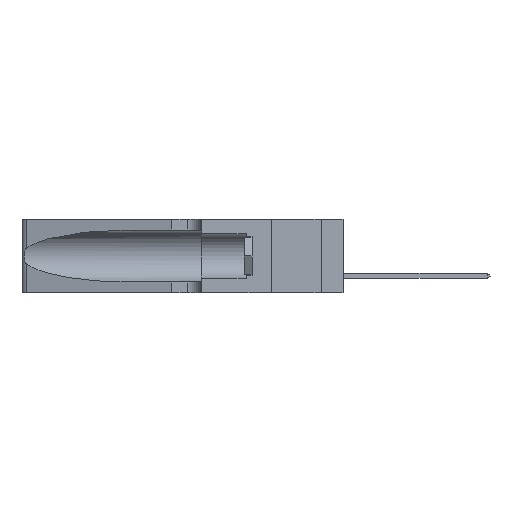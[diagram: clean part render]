
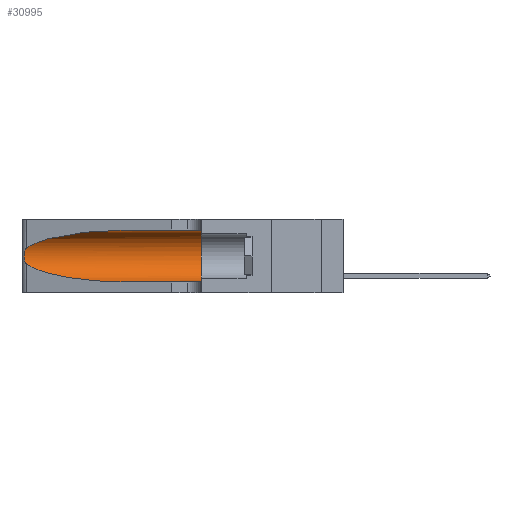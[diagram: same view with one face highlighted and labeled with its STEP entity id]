
A CAD part, left-side view. The second image highlights one B-rep face of the part: STEP entity #30995.
In plain terms, the highlighted cylindrical face has radius 3.308 mm (diameter 6.617 mm), a partial arc.
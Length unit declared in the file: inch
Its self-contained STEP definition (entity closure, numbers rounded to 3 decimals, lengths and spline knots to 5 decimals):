
#220 = CARTESIAN_POINT ( 'NONE',  ( 0.25487, 1.22718, 0.22369 ) ) ;
#691 = CARTESIAN_POINT ( 'NONE',  ( 0.1305, 0.35, 0.185 ) ) ;
#821 = CARTESIAN_POINT ( 'NONE',  ( 0.25789, 1.23486, 0.15765 ) ) ;
#1298 = CARTESIAN_POINT ( 'NONE',  ( 0.25487, 1.22718, 0.14631 ) ) ;
#1674 = CARTESIAN_POINT ( 'NONE',  ( 0.1305, 0.35, 0.05475 ) ) ;
#2868 = CIRCLE ( 'NONE', #6145, 0.13025 ) ;
#4660 = CARTESIAN_POINT ( 'NONE',  ( 0.25787, 1.23484, 0.2124 ) ) ;
#4814 = CARTESIAN_POINT ( 'NONE',  ( 0.26075, 1.23896, 0.178 ) ) ;
#5688 = VECTOR ( 'NONE', #42577, 39.37008 ) ;
#5845 = EDGE_CURVE ( 'NONE', #40393, #30720, #21798, .T. ) ;
#6107 = CARTESIAN_POINT ( 'NONE',  ( 0.1305, 0.72297, 0.05475 ) ) ;
#6145 = AXIS2_PLACEMENT_3D ( 'NONE', #691, #7439, #26365 ) ;
#6199 = CARTESIAN_POINT ( 'NONE',  ( 0.1305, 1.61858, 0.05475 ) ) ;
#6645 = EDGE_CURVE ( 'NONE', #20027, #35176, #32042, .T. ) ;
#7439 = DIRECTION ( 'NONE',  ( 0., 1., 0. ) ) ;
#8121 = DIRECTION ( 'NONE',  ( 0., 0., -1. ) ) ;
#8337 = ORIENTED_EDGE ( 'NONE', *, *, #5845, .T. ) ;
#8373 = CARTESIAN_POINT ( 'NONE',  ( 0.25639, 1.23184, 0.21858 ) ) ;
#9470 = EDGE_CURVE ( 'NONE', #30720, #21175, #28301, .T. ) ;
#10138 = CARTESIAN_POINT ( 'NONE',  ( 0.25487, 1.22718, 0.14631 ) ) ;
#10263 = EDGE_CURVE ( 'NONE', #20027, #40393, #16214, .T. ) ;
#10413 = EDGE_CURVE ( 'NONE', #35176, #31136, #2868, .T. ) ;
#11972 = DIRECTION ( 'NONE',  ( 0., -1., 0. ) ) ;
#12222 = CARTESIAN_POINT ( 'NONE',  ( 0.26075, 1.23896, 0.19203 ) ) ;
#12375 = CARTESIAN_POINT ( 'NONE',  ( 0.26018, 1.23835, 0.19895 ) ) ;
#13506 = EDGE_LOOP ( 'NONE', ( #20761, #8337, #34533, #29191, #28066, #44213 ) ) ;
#16214 =( BOUNDED_CURVE ( )  B_SPLINE_CURVE ( 3, ( #42742, #20967, #28691, #17423 ),
 .UNSPECIFIED., .F., .F. ) 
 B_SPLINE_CURVE_WITH_KNOTS ( ( 4, 4 ),
 ( 1.5708, 2.84003 ),
 .UNSPECIFIED. ) 
 CURVE ( )  GEOMETRIC_REPRESENTATION_ITEM ( )  RATIONAL_B_SPLINE_CURVE ( ( 1., 0.87, 0.87, 1. ) ) 
 REPRESENTATION_ITEM ( '' )  );
#17225 = CARTESIAN_POINT ( 'NONE',  ( 0.1305, 0.35, 0.31525 ) ) ;
#17423 = CARTESIAN_POINT ( 'NONE',  ( 0.25487, 1.22718, 0.22369 ) ) ;
#17577 = CARTESIAN_POINT ( 'NONE',  ( 0.1305, 0.72297, 0.31525 ) ) ;
#20027 = VERTEX_POINT ( 'NONE', #17577 ) ;
#20554 = CARTESIAN_POINT ( 'NONE',  ( 0.2373, 1.15595, 0.08982 ) ) ;
#20761 = ORIENTED_EDGE ( 'NONE', *, *, #10263, .T. ) ;
#20967 = CARTESIAN_POINT ( 'NONE',  ( 0.18966, 0.96281, 0.31525 ) ) ;
#21175 = VERTEX_POINT ( 'NONE', #41529 ) ;
#21798 = B_SPLINE_CURVE_WITH_KNOTS ( 'NONE', 3,
 ( #23424, #34202, #8373, #4660, #45061, #12375, #12222, #4814, #38177, #26821, #821, #37521, #41678, #1298 ),
 .UNSPECIFIED., .F., .F.,
 ( 4, 2, 2, 2, 2, 2, 4 ),
 ( 0., 0.00027, 0.00053, 0.00107, 0.0016, 0.00187, 0.00214 ),
 .UNSPECIFIED. ) ;
#22219 = CARTESIAN_POINT ( 'NONE',  ( 0.1305, 1.61858, 0.185 ) ) ;
#23167 = FACE_OUTER_BOUND ( 'NONE', #13506, .T. ) ;
#23424 = CARTESIAN_POINT ( 'NONE',  ( 0.25487, 1.22718, 0.22369 ) ) ;
#26268 = VECTOR ( 'NONE', #38761, 39.37008 ) ;
#26365 = DIRECTION ( 'NONE',  ( 0., 0., 1. ) ) ;
#26821 = CARTESIAN_POINT ( 'NONE',  ( 0.25856, 1.23593, 0.16098 ) ) ;
#28066 = ORIENTED_EDGE ( 'NONE', *, *, #10413, .F. ) ;
#28301 =( BOUNDED_CURVE ( )  B_SPLINE_CURVE ( 3, ( #10138, #20554, #46183, #6107 ),
 .UNSPECIFIED., .F., .F. ) 
 B_SPLINE_CURVE_WITH_KNOTS ( ( 4, 4 ),
 ( 3.44316, 4.71239 ),
 .UNSPECIFIED. ) 
 CURVE ( )  GEOMETRIC_REPRESENTATION_ITEM ( )  RATIONAL_B_SPLINE_CURVE ( ( 1., 0.87, 0.87, 1. ) ) 
 REPRESENTATION_ITEM ( '' )  );
#28691 = CARTESIAN_POINT ( 'NONE',  ( 0.2373, 1.15595, 0.28018 ) ) ;
#29191 = ORIENTED_EDGE ( 'NONE', *, *, #40890, .T. ) ;
#30720 = VERTEX_POINT ( 'NONE', #31916 ) ;
#30995 = ADVANCED_FACE ( 'NONE', ( #23167 ), #43187, .F. ) ;
#31136 = VERTEX_POINT ( 'NONE', #1674 ) ;
#31916 = CARTESIAN_POINT ( 'NONE',  ( 0.25487, 1.22718, 0.14631 ) ) ;
#32042 = LINE ( 'NONE', #42106, #26268 ) ;
#33736 = AXIS2_PLACEMENT_3D ( 'NONE', #22219, #11972, #8121 ) ;
#34202 = CARTESIAN_POINT ( 'NONE',  ( 0.25555, 1.22994, 0.2215 ) ) ;
#34533 = ORIENTED_EDGE ( 'NONE', *, *, #9470, .T. ) ;
#35176 = VERTEX_POINT ( 'NONE', #17225 ) ;
#37521 = CARTESIAN_POINT ( 'NONE',  ( 0.25639, 1.23186, 0.15144 ) ) ;
#38177 = CARTESIAN_POINT ( 'NONE',  ( 0.26017, 1.23833, 0.17102 ) ) ;
#38761 = DIRECTION ( 'NONE',  ( 0., -1., 0. ) ) ;
#40393 = VERTEX_POINT ( 'NONE', #220 ) ;
#40890 = EDGE_CURVE ( 'NONE', #21175, #31136, #44719, .T. ) ;
#41529 = CARTESIAN_POINT ( 'NONE',  ( 0.1305, 0.72297, 0.05475 ) ) ;
#41678 = CARTESIAN_POINT ( 'NONE',  ( 0.25555, 1.22993, 0.14849 ) ) ;
#42106 = CARTESIAN_POINT ( 'NONE',  ( 0.1305, 1.61858, 0.31525 ) ) ;
#42577 = DIRECTION ( 'NONE',  ( 0., -1., 0. ) ) ;
#42742 = CARTESIAN_POINT ( 'NONE',  ( 0.1305, 0.72297, 0.31525 ) ) ;
#43187 = CYLINDRICAL_SURFACE ( 'NONE', #33736, 0.13025 ) ;
#44213 = ORIENTED_EDGE ( 'NONE', *, *, #6645, .F. ) ;
#44719 = LINE ( 'NONE', #6199, #5688 ) ;
#45061 = CARTESIAN_POINT ( 'NONE',  ( 0.25854, 1.2359, 0.20912 ) ) ;
#46183 = CARTESIAN_POINT ( 'NONE',  ( 0.18966, 0.96281, 0.05475 ) ) ;
